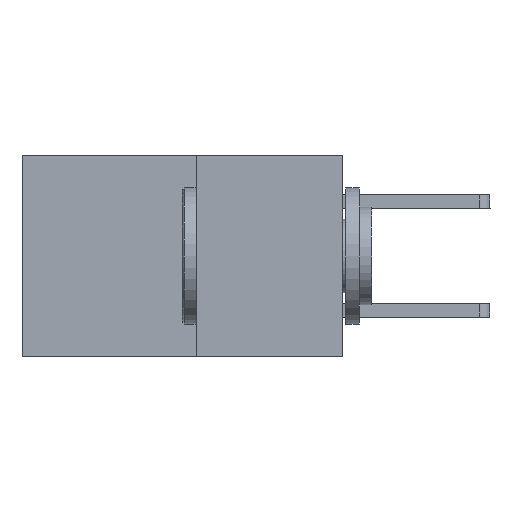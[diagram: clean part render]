
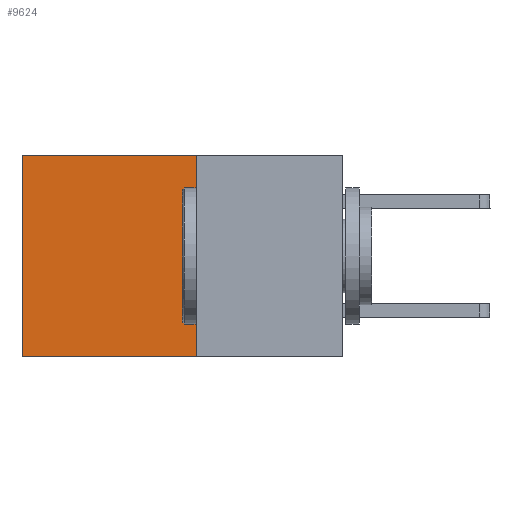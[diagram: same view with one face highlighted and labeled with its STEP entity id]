
A CAD part, left-side view. The second image highlights one B-rep face of the part: STEP entity #9624.
In plain terms, the highlighted planar face has unit normal (-1, 0, 0).
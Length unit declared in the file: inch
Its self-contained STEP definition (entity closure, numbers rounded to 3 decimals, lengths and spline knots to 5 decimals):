
#74 = LINE ( 'NONE', #1403, #8563 ) ;
#643 = VERTEX_POINT ( 'NONE', #9537 ) ;
#672 = LINE ( 'NONE', #5364, #6744 ) ;
#1334 = VERTEX_POINT ( 'NONE', #5332 ) ;
#1403 = CARTESIAN_POINT ( 'NONE',  ( 0.277, 0.27, -0.37 ) ) ;
#1458 = EDGE_CURVE ( 'NONE', #1334, #8197, #672, .T. ) ;
#1493 = PLANE ( 'NONE',  #8048 ) ;
#2314 = DIRECTION ( 'NONE',  ( 1., 0., 0. ) ) ;
#2812 = CARTESIAN_POINT ( 'NONE',  ( 0.277, 0.27, 0. ) ) ;
#3052 = DIRECTION ( 'NONE',  ( 0., 1., 0. ) ) ;
#4073 = DIRECTION ( 'NONE',  ( 0., 1., 0. ) ) ;
#4215 = EDGE_CURVE ( 'NONE', #643, #8197, #74, .T. ) ;
#4942 = EDGE_CURVE ( 'NONE', #7883, #1334, #8671, .T. ) ;
#5006 = CARTESIAN_POINT ( 'NONE',  ( 0.277, 0.27, -0.37 ) ) ;
#5037 = CARTESIAN_POINT ( 'NONE',  ( 0.277, 0.27, 0. ) ) ;
#5332 = CARTESIAN_POINT ( 'NONE',  ( 0.277, 0.59, 0. ) ) ;
#5364 = CARTESIAN_POINT ( 'NONE',  ( 0.277, 0.59, -0.37 ) ) ;
#5620 = CARTESIAN_POINT ( 'NONE',  ( 0.277, 0.59, -0.37 ) ) ;
#5845 = DIRECTION ( 'NONE',  ( 0., 0., -1. ) ) ;
#6040 = VECTOR ( 'NONE', #5845, 39.37008 ) ;
#6307 = VECTOR ( 'NONE', #4073, 39.37008 ) ;
#6432 = ORIENTED_EDGE ( 'NONE', *, *, #4215, .F. ) ;
#6744 = VECTOR ( 'NONE', #8736, 39.37008 ) ;
#7075 = ORIENTED_EDGE ( 'NONE', *, *, #4942, .T. ) ;
#7081 = ORIENTED_EDGE ( 'NONE', *, *, #1458, .T. ) ;
#7219 = CARTESIAN_POINT ( 'NONE',  ( 0.277, 0.27, -0.37 ) ) ;
#7590 = EDGE_CURVE ( 'NONE', #7883, #643, #8151, .T. ) ;
#7883 = VERTEX_POINT ( 'NONE', #2812 ) ;
#8031 = DIRECTION ( 'NONE',  ( 0., 0., -1. ) ) ;
#8048 = AXIS2_PLACEMENT_3D ( 'NONE', #7219, #2314, #8031 ) ;
#8151 = LINE ( 'NONE', #5006, #6040 ) ;
#8197 = VERTEX_POINT ( 'NONE', #5620 ) ;
#8354 = FACE_OUTER_BOUND ( 'NONE', #10215, .T. ) ;
#8563 = VECTOR ( 'NONE', #3052, 39.37008 ) ;
#8639 = ORIENTED_EDGE ( 'NONE', *, *, #7590, .F. ) ;
#8671 = LINE ( 'NONE', #5037, #6307 ) ;
#8736 = DIRECTION ( 'NONE',  ( 0., 0., -1. ) ) ;
#9537 = CARTESIAN_POINT ( 'NONE',  ( 0.277, 0.27, -0.37 ) ) ;
#9624 = ADVANCED_FACE ( 'NONE', ( #8354 ), #1493, .F. ) ;
#10215 = EDGE_LOOP ( 'NONE', ( #7081, #6432, #8639, #7075 ) ) ;
